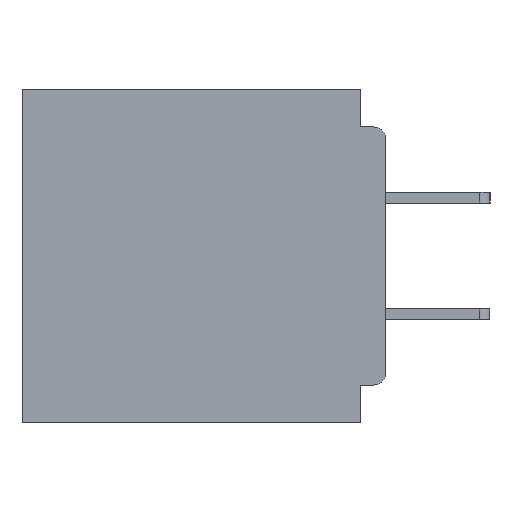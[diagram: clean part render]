
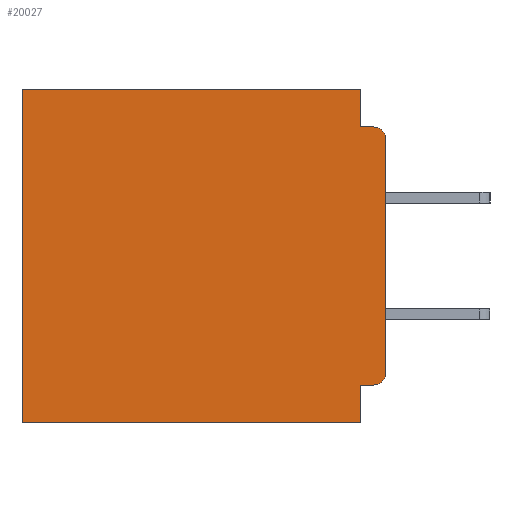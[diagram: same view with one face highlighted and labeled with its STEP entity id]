
A CAD part, left-side view. The second image highlights one B-rep face of the part: STEP entity #20027.
In plain terms, the highlighted planar face has unit normal (-1, 0, 0).
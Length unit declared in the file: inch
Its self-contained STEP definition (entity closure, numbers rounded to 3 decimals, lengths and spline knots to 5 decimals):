
#65 = ORIENTED_EDGE ( 'NONE', *, *, #21503, .F. ) ;
#585 = VERTEX_POINT ( 'NONE', #43065 ) ;
#830 = DIRECTION ( 'NONE',  ( 0., 0., -1. ) ) ;
#1271 = LINE ( 'NONE', #3644, #18704 ) ;
#1292 = FACE_OUTER_BOUND ( 'NONE', #24531, .T. ) ;
#1337 = DIRECTION ( 'NONE',  ( 0., 1., 0. ) ) ;
#3643 = CARTESIAN_POINT ( 'NONE',  ( 0.3, 0.031, -0.4 ) ) ;
#3644 = CARTESIAN_POINT ( 'NONE',  ( 0.3, 0., -0.045 ) ) ;
#4232 = VERTEX_POINT ( 'NONE', #18029 ) ;
#4630 = CARTESIAN_POINT ( 'NONE',  ( 0.3, 0.031, 0. ) ) ;
#4942 = ORIENTED_EDGE ( 'NONE', *, *, #9341, .T. ) ;
#5168 = ORIENTED_EDGE ( 'NONE', *, *, #23263, .F. ) ;
#5503 = ORIENTED_EDGE ( 'NONE', *, *, #29937, .F. ) ;
#5579 = VERTEX_POINT ( 'NONE', #21546 ) ;
#6202 = CARTESIAN_POINT ( 'NONE',  ( 0.3, 0., -0.355 ) ) ;
#6340 = CARTESIAN_POINT ( 'NONE',  ( 0.3, 0.437, 0. ) ) ;
#6755 = EDGE_CURVE ( 'NONE', #11411, #5579, #27093, .T. ) ;
#6842 = CIRCLE ( 'NONE', #25472, 0.015 ) ;
#6942 = VECTOR ( 'NONE', #23296, 39.37008 ) ;
#7429 = LINE ( 'NONE', #11508, #24932 ) ;
#7808 = VERTEX_POINT ( 'NONE', #21261 ) ;
#8777 = ORIENTED_EDGE ( 'NONE', *, *, #6755, .F. ) ;
#9341 = EDGE_CURVE ( 'NONE', #4232, #7808, #21371, .T. ) ;
#10002 = LINE ( 'NONE', #25730, #18203 ) ;
#10476 = DIRECTION ( 'NONE',  ( 0., 0., -1. ) ) ;
#10627 = DIRECTION ( 'NONE',  ( 0., -1., 0. ) ) ;
#11411 = VERTEX_POINT ( 'NONE', #40753 ) ;
#11508 = CARTESIAN_POINT ( 'NONE',  ( 0.3, 0.031, 0. ) ) ;
#11584 = ORIENTED_EDGE ( 'NONE', *, *, #32863, .F. ) ;
#12682 = ORIENTED_EDGE ( 'NONE', *, *, #30761, .F. ) ;
#12826 = DIRECTION ( 'NONE',  ( 1., 0., 0. ) ) ;
#12891 = EDGE_CURVE ( 'NONE', #21234, #43214, #6842, .T. ) ;
#12912 = CARTESIAN_POINT ( 'NONE',  ( 0.3, 0.015, -0.34 ) ) ;
#13416 = VECTOR ( 'NONE', #10476, 39.37008 ) ;
#14119 = EDGE_CURVE ( 'NONE', #28528, #32196, #10002, .T. ) ;
#15086 = CARTESIAN_POINT ( 'NONE',  ( 0.3, 0., -0.06 ) ) ;
#15874 = CARTESIAN_POINT ( 'NONE',  ( 0.3, 0., -0.4 ) ) ;
#16446 = DIRECTION ( 'NONE',  ( 0., 0., -1. ) ) ;
#17347 = LINE ( 'NONE', #33751, #6942 ) ;
#17454 = ORIENTED_EDGE ( 'NONE', *, *, #39736, .T. ) ;
#18029 = CARTESIAN_POINT ( 'NONE',  ( 0.3, 0.015, -0.355 ) ) ;
#18203 = VECTOR ( 'NONE', #1337, 39.37008 ) ;
#18515 = DIRECTION ( 'NONE',  ( 0., 0., -1. ) ) ;
#18704 = VECTOR ( 'NONE', #10627, 39.37008 ) ;
#19374 = DIRECTION ( 'NONE',  ( 0., 1., 0. ) ) ;
#20027 = ADVANCED_FACE ( 'NONE', ( #1292 ), #33808, .F. ) ;
#21234 = VERTEX_POINT ( 'NONE', #15086 ) ;
#21261 = CARTESIAN_POINT ( 'NONE',  ( 0.3, 0., -0.34 ) ) ;
#21371 = CIRCLE ( 'NONE', #42962, 0.015 ) ;
#21503 = EDGE_CURVE ( 'NONE', #4232, #27933, #32886, .T. ) ;
#21546 = CARTESIAN_POINT ( 'NONE',  ( 0.3, 0.437, -0.4 ) ) ;
#21673 = DIRECTION ( 'NONE',  ( -1., 0., 0. ) ) ;
#21819 = VECTOR ( 'NONE', #35601, 39.37008 ) ;
#23263 = EDGE_CURVE ( 'NONE', #21234, #7808, #17347, .T. ) ;
#23296 = DIRECTION ( 'NONE',  ( 0., 0., -1. ) ) ;
#24004 = CARTESIAN_POINT ( 'NONE',  ( 0.3, 0.015, -0.045 ) ) ;
#24531 = EDGE_LOOP ( 'NONE', ( #5168, #38720, #11584, #12682, #35240, #17454, #8777, #5503, #65, #4942 ) ) ;
#24932 = VECTOR ( 'NONE', #18515, 39.37008 ) ;
#25472 = AXIS2_PLACEMENT_3D ( 'NONE', #42581, #21673, #830 ) ;
#25711 = VECTOR ( 'NONE', #30696, 39.37008 ) ;
#25730 = CARTESIAN_POINT ( 'NONE',  ( 0.3, 0., 0. ) ) ;
#27093 = LINE ( 'NONE', #15874, #35271 ) ;
#27933 = VERTEX_POINT ( 'NONE', #39334 ) ;
#28528 = VERTEX_POINT ( 'NONE', #4630 ) ;
#29937 = EDGE_CURVE ( 'NONE', #27933, #11411, #30975, .T. ) ;
#30696 = DIRECTION ( 'NONE',  ( 0., 1., 0. ) ) ;
#30761 = EDGE_CURVE ( 'NONE', #28528, #585, #7429, .T. ) ;
#30975 = LINE ( 'NONE', #3643, #13416 ) ;
#32115 = CARTESIAN_POINT ( 'NONE',  ( 0.3, 0.437, -0.4 ) ) ;
#32196 = VERTEX_POINT ( 'NONE', #6340 ) ;
#32863 = EDGE_CURVE ( 'NONE', #585, #43214, #1271, .T. ) ;
#32886 = LINE ( 'NONE', #6202, #25711 ) ;
#33751 = CARTESIAN_POINT ( 'NONE',  ( 0.3, 0., -0.4 ) ) ;
#33808 = PLANE ( 'NONE',  #35066 ) ;
#35066 = AXIS2_PLACEMENT_3D ( 'NONE', #44090, #12826, #37295 ) ;
#35240 = ORIENTED_EDGE ( 'NONE', *, *, #14119, .T. ) ;
#35271 = VECTOR ( 'NONE', #19374, 39.37008 ) ;
#35601 = DIRECTION ( 'NONE',  ( 0., 0., -1. ) ) ;
#37295 = DIRECTION ( 'NONE',  ( 0., 0., -1. ) ) ;
#37368 = DIRECTION ( 'NONE',  ( -1., 0., 0. ) ) ;
#38720 = ORIENTED_EDGE ( 'NONE', *, *, #12891, .T. ) ;
#39334 = CARTESIAN_POINT ( 'NONE',  ( 0.3, 0.031, -0.355 ) ) ;
#39736 = EDGE_CURVE ( 'NONE', #32196, #5579, #40416, .T. ) ;
#40416 = LINE ( 'NONE', #32115, #21819 ) ;
#40753 = CARTESIAN_POINT ( 'NONE',  ( 0.3, 0.031, -0.4 ) ) ;
#42581 = CARTESIAN_POINT ( 'NONE',  ( 0.3, 0.015, -0.06 ) ) ;
#42962 = AXIS2_PLACEMENT_3D ( 'NONE', #12912, #37368, #16446 ) ;
#43065 = CARTESIAN_POINT ( 'NONE',  ( 0.3, 0.031, -0.045 ) ) ;
#43214 = VERTEX_POINT ( 'NONE', #24004 ) ;
#44090 = CARTESIAN_POINT ( 'NONE',  ( 0.3, 0., -0.4 ) ) ;
